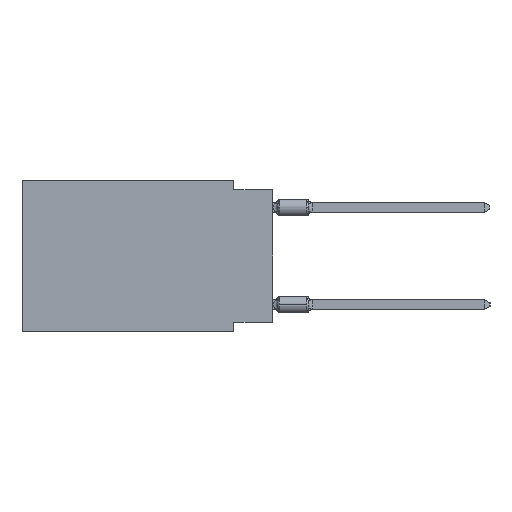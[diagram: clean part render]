
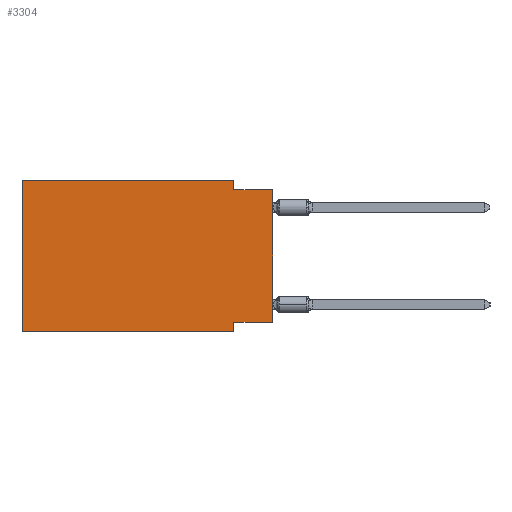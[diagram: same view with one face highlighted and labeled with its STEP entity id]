
A CAD part, left-side view. The second image highlights one B-rep face of the part: STEP entity #3304.
In plain terms, the highlighted planar face has unit normal (-1, 0, 0).
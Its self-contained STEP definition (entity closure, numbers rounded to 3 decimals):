
#771 = CARTESIAN_POINT ( 'NONE',  ( 0., 2.54, -9.906 ) ) ;
#810 = CARTESIAN_POINT ( 'NONE',  ( 0., 0., -0.635 ) ) ;
#1207 = DIRECTION ( 'NONE',  ( 0., -1., 0. ) ) ;
#1428 = VERTEX_POINT ( 'NONE', #20399 ) ;
#1917 = CARTESIAN_POINT ( 'NONE',  ( 0., 0., 0. ) ) ;
#2566 = VECTOR ( 'NONE', #18611, 1000. ) ;
#3304 = ADVANCED_FACE ( 'NONE', ( #27489 ), #6840, .F. ) ;
#3521 = LINE ( 'NONE', #32580, #7677 ) ;
#3748 = VERTEX_POINT ( 'NONE', #11794 ) ;
#3789 = LINE ( 'NONE', #24778, #14645 ) ;
#5276 = CARTESIAN_POINT ( 'NONE',  ( 0., 2.54, -9.271 ) ) ;
#6840 = PLANE ( 'NONE',  #17278 ) ;
#7136 = ORIENTED_EDGE ( 'NONE', *, *, #19712, .F. ) ;
#7677 = VECTOR ( 'NONE', #30348, 1000. ) ;
#8305 = CARTESIAN_POINT ( 'NONE',  ( 0., 2.54, -9.906 ) ) ;
#8421 = VERTEX_POINT ( 'NONE', #27474 ) ;
#8630 = VERTEX_POINT ( 'NONE', #771 ) ;
#9156 = ORIENTED_EDGE ( 'NONE', *, *, #31009, .T. ) ;
#9190 = EDGE_CURVE ( 'NONE', #3748, #8630, #3789, .T. ) ;
#9930 = ORIENTED_EDGE ( 'NONE', *, *, #24599, .F. ) ;
#10400 = VECTOR ( 'NONE', #26198, 1000. ) ;
#10517 = VECTOR ( 'NONE', #22903, 1000. ) ;
#10679 = CARTESIAN_POINT ( 'NONE',  ( 0., 16.383, 0. ) ) ;
#11794 = CARTESIAN_POINT ( 'NONE',  ( 0., 16.383, -9.906 ) ) ;
#11989 = VERTEX_POINT ( 'NONE', #5276 ) ;
#12078 = CARTESIAN_POINT ( 'NONE',  ( 0., 2.54, 0. ) ) ;
#12621 = VERTEX_POINT ( 'NONE', #32396 ) ;
#13619 = ORIENTED_EDGE ( 'NONE', *, *, #33675, .F. ) ;
#14076 = EDGE_CURVE ( 'NONE', #1428, #26522, #22933, .T. ) ;
#14222 = ORIENTED_EDGE ( 'NONE', *, *, #14076, .F. ) ;
#14489 = ORIENTED_EDGE ( 'NONE', *, *, #9190, .T. ) ;
#14515 = DIRECTION ( 'NONE',  ( 0., -1., 0. ) ) ;
#14593 = CARTESIAN_POINT ( 'NONE',  ( 0., 16.383, 0. ) ) ;
#14645 = VECTOR ( 'NONE', #1207, 1000. ) ;
#14670 = ORIENTED_EDGE ( 'NONE', *, *, #28521, .F. ) ;
#14733 = VECTOR ( 'NONE', #14515, 1000. ) ;
#14944 = DIRECTION ( 'NONE',  ( 0., 0., -1. ) ) ;
#15383 = DIRECTION ( 'NONE',  ( 0., -1., 0. ) ) ;
#17278 = AXIS2_PLACEMENT_3D ( 'NONE', #14593, #20078, #14944 ) ;
#17703 = CARTESIAN_POINT ( 'NONE',  ( 0., 16.383, 0. ) ) ;
#18611 = DIRECTION ( 'NONE',  ( 0., 0., 1. ) ) ;
#18638 = LINE ( 'NONE', #8305, #10400 ) ;
#19712 = EDGE_CURVE ( 'NONE', #29204, #12621, #29651, .T. ) ;
#19905 = ORIENTED_EDGE ( 'NONE', *, *, #29380, .F. ) ;
#20078 = DIRECTION ( 'NONE',  ( 1., 0., 0. ) ) ;
#20399 = CARTESIAN_POINT ( 'NONE',  ( 0., 2.54, -0.635 ) ) ;
#20476 = LINE ( 'NONE', #12078, #27317 ) ;
#20493 = LINE ( 'NONE', #1917, #10517 ) ;
#21387 = EDGE_LOOP ( 'NONE', ( #9156, #14222, #9930, #7136, #13619, #14489, #14670, #19905 ) ) ;
#22234 = CARTESIAN_POINT ( 'NONE',  ( 0., 16.383, 0. ) ) ;
#22903 = DIRECTION ( 'NONE',  ( 0., 0., 1. ) ) ;
#22933 = LINE ( 'NONE', #33422, #27724 ) ;
#24599 = EDGE_CURVE ( 'NONE', #12621, #1428, #20476, .T. ) ;
#24778 = CARTESIAN_POINT ( 'NONE',  ( 0., 16.383, -9.906 ) ) ;
#26198 = DIRECTION ( 'NONE',  ( 0., 0., -1. ) ) ;
#26522 = VERTEX_POINT ( 'NONE', #810 ) ;
#27317 = VECTOR ( 'NONE', #30951, 1000. ) ;
#27474 = CARTESIAN_POINT ( 'NONE',  ( 0., 0., -9.271 ) ) ;
#27489 = FACE_OUTER_BOUND ( 'NONE', #21387, .T. ) ;
#27724 = VECTOR ( 'NONE', #15383, 1000. ) ;
#28521 = EDGE_CURVE ( 'NONE', #11989, #8630, #18638, .T. ) ;
#29204 = VERTEX_POINT ( 'NONE', #17703 ) ;
#29380 = EDGE_CURVE ( 'NONE', #8421, #11989, #3521, .T. ) ;
#29651 = LINE ( 'NONE', #22234, #14733 ) ;
#30348 = DIRECTION ( 'NONE',  ( 0., 1., 0. ) ) ;
#30951 = DIRECTION ( 'NONE',  ( 0., 0., -1. ) ) ;
#31009 = EDGE_CURVE ( 'NONE', #8421, #26522, #20493, .T. ) ;
#31991 = LINE ( 'NONE', #10679, #2566 ) ;
#32396 = CARTESIAN_POINT ( 'NONE',  ( 0., 2.54, 0. ) ) ;
#32580 = CARTESIAN_POINT ( 'NONE',  ( 0., 0., -9.271 ) ) ;
#33422 = CARTESIAN_POINT ( 'NONE',  ( 0., 0., -0.635 ) ) ;
#33675 = EDGE_CURVE ( 'NONE', #3748, #29204, #31991, .T. ) ;
